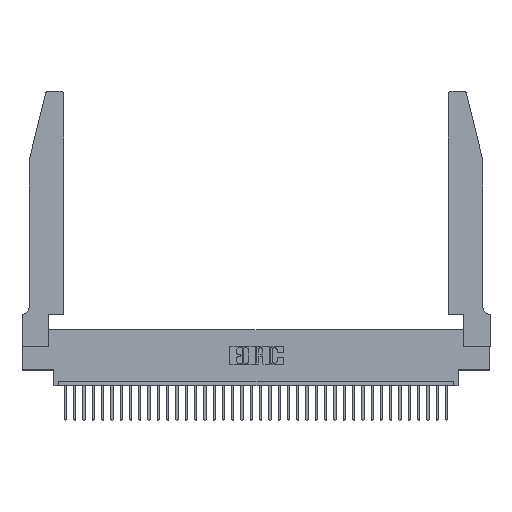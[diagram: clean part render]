
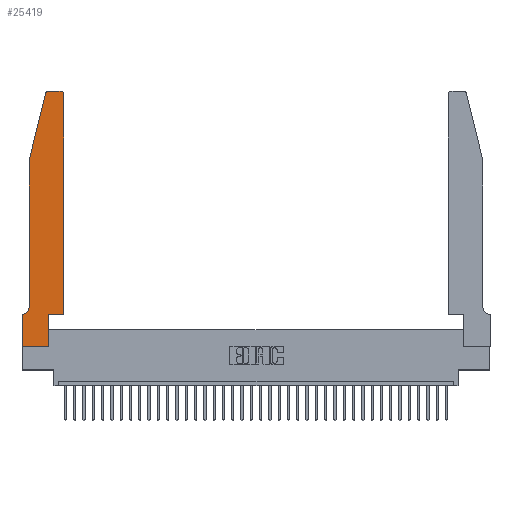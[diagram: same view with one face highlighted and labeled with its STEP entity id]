
A CAD part, top view. The second image highlights one B-rep face of the part: STEP entity #25419.
In plain terms, the highlighted planar face has unit normal (0, 0, 1).
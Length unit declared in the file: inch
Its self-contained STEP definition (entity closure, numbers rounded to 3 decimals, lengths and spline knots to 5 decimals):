
#777 = CARTESIAN_POINT ( 'NONE',  ( 0.0755, 2., 0.37 ) ) ;
#1209 = VERTEX_POINT ( 'NONE', #23298 ) ;
#1685 = EDGE_CURVE ( 'NONE', #29856, #35666, #13352, .T. ) ;
#1916 = DIRECTION ( 'NONE',  ( 1., 0., 0. ) ) ;
#2762 = VECTOR ( 'NONE', #28416, 39.37008 ) ;
#3010 = CARTESIAN_POINT ( 'NONE',  ( 0.4505, 0.35, 0.37 ) ) ;
#3926 = ORIENTED_EDGE ( 'NONE', *, *, #17595, .T. ) ;
#4044 = CARTESIAN_POINT ( 'NONE',  ( 0.0055, 0.42, 0.37 ) ) ;
#4310 = FACE_OUTER_BOUND ( 'NONE', #30267, .T. ) ;
#4576 = CARTESIAN_POINT ( 'NONE',  ( 0.4505, 0.35, 0.37 ) ) ;
#4663 = DIRECTION ( 'NONE',  ( 0., -1., 0. ) ) ;
#4969 = LINE ( 'NONE', #20030, #2762 ) ;
#5161 = CARTESIAN_POINT ( 'NONE',  ( 0.0755, 0.42, 0.37 ) ) ;
#5540 = ORIENTED_EDGE ( 'NONE', *, *, #18201, .T. ) ;
#5574 = CARTESIAN_POINT ( 'NONE',  ( 0.25487, 2.72718, 0.37 ) ) ;
#5771 = ORIENTED_EDGE ( 'NONE', *, *, #31081, .T. ) ;
#5965 = EDGE_CURVE ( 'NONE', #26566, #29593, #12957, .T. ) ;
#6902 = VERTEX_POINT ( 'NONE', #5574 ) ;
#7573 = AXIS2_PLACEMENT_3D ( 'NONE', #19168, #22133, #8169 ) ;
#7796 = ORIENTED_EDGE ( 'NONE', *, *, #1685, .T. ) ;
#8052 = CARTESIAN_POINT ( 'NONE',  ( 0.0755, 2., 0.37 ) ) ;
#8089 = CARTESIAN_POINT ( 'NONE',  ( 0.0755, 2., 0.37 ) ) ;
#8169 = DIRECTION ( 'NONE',  ( 1., 0., 0. ) ) ;
#8518 = VERTEX_POINT ( 'NONE', #777 ) ;
#9321 = DIRECTION ( 'NONE',  ( 0., 0., 1. ) ) ;
#9433 = CARTESIAN_POINT ( 'NONE',  ( 0.0055, 0.35, 0.37 ) ) ;
#10064 = VECTOR ( 'NONE', #35960, 39.37008 ) ;
#10461 = CARTESIAN_POINT ( 'NONE',  ( 0.284, 2.75, 0.37 ) ) ;
#11144 = PLANE ( 'NONE',  #7573 ) ;
#11654 = DIRECTION ( 'NONE',  ( 0., 1., 0. ) ) ;
#11740 = EDGE_CURVE ( 'NONE', #14886, #16947, #16744, .T. ) ;
#11799 = VECTOR ( 'NONE', #27163, 39.37008 ) ;
#12254 = VECTOR ( 'NONE', #16765, 39.37008 ) ;
#12536 = EDGE_CURVE ( 'NONE', #35666, #15113, #36100, .T. ) ;
#12860 = AXIS2_PLACEMENT_3D ( 'NONE', #28938, #9321, #17605 ) ;
#12957 = CIRCLE ( 'NONE', #25849, 0.07 ) ;
#13352 = CIRCLE ( 'NONE', #35178, 0.03 ) ;
#13511 = VECTOR ( 'NONE', #4663, 39.37008 ) ;
#13822 = ORIENTED_EDGE ( 'NONE', *, *, #33411, .T. ) ;
#13926 = LINE ( 'NONE', #35757, #13511 ) ;
#14572 = VECTOR ( 'NONE', #11654, 39.37008 ) ;
#14886 = VERTEX_POINT ( 'NONE', #24978 ) ;
#14922 = DIRECTION ( 'NONE',  ( -1., 0., 0. ) ) ;
#15113 = VERTEX_POINT ( 'NONE', #10461 ) ;
#15353 = LINE ( 'NONE', #27098, #10064 ) ;
#15604 = ORIENTED_EDGE ( 'NONE', *, *, #5965, .T. ) ;
#16744 = LINE ( 'NONE', #26573, #18536 ) ;
#16765 = DIRECTION ( 'NONE',  ( -1., 0., 0. ) ) ;
#16947 = VERTEX_POINT ( 'NONE', #34017 ) ;
#17512 = EDGE_CURVE ( 'NONE', #8518, #26566, #27426, .T. ) ;
#17595 = EDGE_CURVE ( 'NONE', #22846, #29856, #20803, .T. ) ;
#17605 = DIRECTION ( 'NONE',  ( 1., 0., 0. ) ) ;
#18170 = ORIENTED_EDGE ( 'NONE', *, *, #29479, .T. ) ;
#18201 = EDGE_CURVE ( 'NONE', #6902, #8518, #35728, .T. ) ;
#18428 = LINE ( 'NONE', #4576, #11799 ) ;
#18536 = VECTOR ( 'NONE', #1916, 39.37008 ) ;
#19168 = CARTESIAN_POINT ( 'NONE',  ( 0., 0.35, 0.37 ) ) ;
#19591 = DIRECTION ( 'NONE',  ( 1., 0., 0. ) ) ;
#19714 = CARTESIAN_POINT ( 'NONE',  ( 0.2605, 2.75, 0.37 ) ) ;
#20030 = CARTESIAN_POINT ( 'NONE',  ( 0.0755, 0.35, 0.37 ) ) ;
#20803 = LINE ( 'NONE', #3010, #14572 ) ;
#21701 = VECTOR ( 'NONE', #25242, 39.37008 ) ;
#22133 = DIRECTION ( 'NONE',  ( 0., 0., 1. ) ) ;
#22846 = VERTEX_POINT ( 'NONE', #29443 ) ;
#23298 = CARTESIAN_POINT ( 'NONE',  ( 0., 0.35, 0.37 ) ) ;
#24202 = VERTEX_POINT ( 'NONE', #27527 ) ;
#24769 = ORIENTED_EDGE ( 'NONE', *, *, #12536, .T. ) ;
#24978 = CARTESIAN_POINT ( 'NONE',  ( 0., 0., 0.37 ) ) ;
#25242 = DIRECTION ( 'NONE',  ( 0., -1., 0. ) ) ;
#25419 = ADVANCED_FACE ( 'NONE', ( #4310 ), #11144, .T. ) ;
#25606 = CARTESIAN_POINT ( 'NONE',  ( 0.4505, 2.72, 0.37 ) ) ;
#25849 = AXIS2_PLACEMENT_3D ( 'NONE', #4044, #26291, #14922 ) ;
#26291 = DIRECTION ( 'NONE',  ( 0., 0., -1. ) ) ;
#26566 = VERTEX_POINT ( 'NONE', #5161 ) ;
#26573 = CARTESIAN_POINT ( 'NONE',  ( 0., 0., 0.37 ) ) ;
#27098 = CARTESIAN_POINT ( 'NONE',  ( 0.2865, 0.35, 0.37 ) ) ;
#27163 = DIRECTION ( 'NONE',  ( 1., 0., 0. ) ) ;
#27426 = LINE ( 'NONE', #8089, #21701 ) ;
#27527 = CARTESIAN_POINT ( 'NONE',  ( 0.2865, 0.35, 0.37 ) ) ;
#27892 = CARTESIAN_POINT ( 'NONE',  ( 0.4205, 2.75, 0.37 ) ) ;
#27991 = CIRCLE ( 'NONE', #12860, 0.03 ) ;
#28416 = DIRECTION ( 'NONE',  ( -1., 0., 0. ) ) ;
#28452 = DIRECTION ( 'NONE',  ( 0., 0., 1. ) ) ;
#28938 = CARTESIAN_POINT ( 'NONE',  ( 0.284, 2.72, 0.37 ) ) ;
#29443 = CARTESIAN_POINT ( 'NONE',  ( 0.4505, 0.35, 0.37 ) ) ;
#29479 = EDGE_CURVE ( 'NONE', #15113, #6902, #27991, .T. ) ;
#29593 = VERTEX_POINT ( 'NONE', #9433 ) ;
#29856 = VERTEX_POINT ( 'NONE', #25606 ) ;
#30267 = EDGE_LOOP ( 'NONE', ( #24769, #18170, #5540, #30278, #15604, #5771, #33661, #34685, #13822, #30782, #3926, #7796 ) ) ;
#30278 = ORIENTED_EDGE ( 'NONE', *, *, #17512, .T. ) ;
#30619 = DIRECTION ( 'NONE',  ( -0.239, -0.971, 0. ) ) ;
#30782 = ORIENTED_EDGE ( 'NONE', *, *, #35568, .T. ) ;
#31081 = EDGE_CURVE ( 'NONE', #29593, #1209, #4969, .T. ) ;
#31168 = CARTESIAN_POINT ( 'NONE',  ( 0.4205, 2.72, 0.37 ) ) ;
#33411 = EDGE_CURVE ( 'NONE', #16947, #24202, #15353, .T. ) ;
#33661 = ORIENTED_EDGE ( 'NONE', *, *, #34224, .T. ) ;
#33958 = VECTOR ( 'NONE', #30619, 39.37008 ) ;
#34017 = CARTESIAN_POINT ( 'NONE',  ( 0.2865, 0., 0.37 ) ) ;
#34224 = EDGE_CURVE ( 'NONE', #1209, #14886, #13926, .T. ) ;
#34685 = ORIENTED_EDGE ( 'NONE', *, *, #11740, .T. ) ;
#35178 = AXIS2_PLACEMENT_3D ( 'NONE', #31168, #28452, #19591 ) ;
#35568 = EDGE_CURVE ( 'NONE', #24202, #22846, #18428, .T. ) ;
#35666 = VERTEX_POINT ( 'NONE', #27892 ) ;
#35728 = LINE ( 'NONE', #8052, #33958 ) ;
#35757 = CARTESIAN_POINT ( 'NONE',  ( 0., 0., 0.37 ) ) ;
#35960 = DIRECTION ( 'NONE',  ( 0., 1., 0. ) ) ;
#36100 = LINE ( 'NONE', #19714, #12254 ) ;
